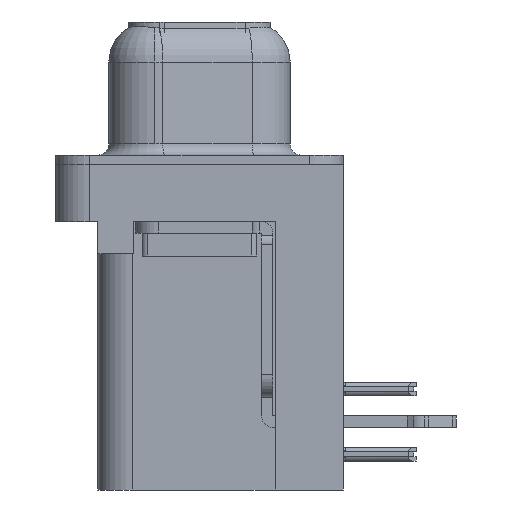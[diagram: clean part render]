
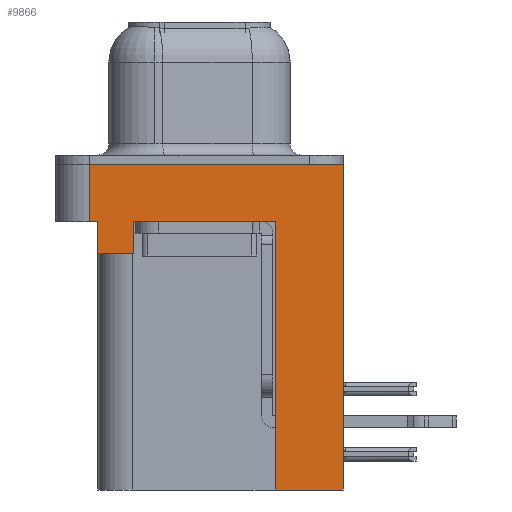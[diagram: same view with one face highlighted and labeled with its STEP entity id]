
A CAD part, left-side view. The second image highlights one B-rep face of the part: STEP entity #9866.
In plain terms, the highlighted planar face has unit normal (-1, 0, 0).
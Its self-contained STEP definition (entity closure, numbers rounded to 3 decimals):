
#662 = ORIENTED_EDGE ( 'NONE', *, *, #22296, .F. ) ;
#975 = CARTESIAN_POINT ( 'NONE',  ( -2.91, -3.295, -14.2 ) ) ;
#1129 = ORIENTED_EDGE ( 'NONE', *, *, #33008, .F. ) ;
#1270 = VECTOR ( 'NONE', #12453, 1000. ) ;
#1343 = EDGE_CURVE ( 'NONE', #36206, #31903, #29630, .T. ) ;
#2132 = LINE ( 'NONE', #27914, #9088 ) ;
#2595 = CARTESIAN_POINT ( 'NONE',  ( -2.91, -6.275, -14.2 ) ) ;
#2701 = EDGE_CURVE ( 'NONE', #25302, #26912, #2132, .T. ) ;
#2779 = CARTESIAN_POINT ( 'NONE',  ( -2.91, -3.295, -14.2 ) ) ;
#3863 = DIRECTION ( 'NONE',  ( 0., 0., 1. ) ) ;
#4467 = LINE ( 'NONE', #21187, #1270 ) ;
#5905 = LINE ( 'NONE', #31322, #26976 ) ;
#6474 = ORIENTED_EDGE ( 'NONE', *, *, #16695, .F. ) ;
#7933 = CARTESIAN_POINT ( 'NONE',  ( -2.91, -3.295, -2.5 ) ) ;
#8213 = CARTESIAN_POINT ( 'NONE',  ( -2.91, 4.775, -2.5 ) ) ;
#8219 = DIRECTION ( 'NONE',  ( 0., 0., 1. ) ) ;
#8306 = CARTESIAN_POINT ( 'NONE',  ( -2.91, 4.425, -3.9 ) ) ;
#8518 = ORIENTED_EDGE ( 'NONE', *, *, #31069, .F. ) ;
#8621 = DIRECTION ( 'NONE',  ( 0., 0., 1. ) ) ;
#8640 = EDGE_LOOP ( 'NONE', ( #11275, #8518, #35854, #1129, #662, #28178, #12209, #31163, #6474, #33613 ) ) ;
#8813 = LINE ( 'NONE', #14006, #20465 ) ;
#8950 = LINE ( 'NONE', #975, #25803 ) ;
#8978 = DIRECTION ( 'NONE',  ( 0., 0., 1. ) ) ;
#9088 = VECTOR ( 'NONE', #36262, 1000. ) ;
#9105 = VERTEX_POINT ( 'NONE', #32673 ) ;
#9159 = EDGE_CURVE ( 'NONE', #9105, #36573, #4467, .T. ) ;
#9362 = VECTOR ( 'NONE', #3863, 1000. ) ;
#9866 = ADVANCED_FACE ( 'NONE', ( #32183 ), #26425, .T. ) ;
#10618 = VERTEX_POINT ( 'NONE', #2779 ) ;
#11275 = ORIENTED_EDGE ( 'NONE', *, *, #1343, .F. ) ;
#12209 = ORIENTED_EDGE ( 'NONE', *, *, #9159, .T. ) ;
#12453 = DIRECTION ( 'NONE',  ( 0., -1., 0. ) ) ;
#12659 = VECTOR ( 'NONE', #35088, 1000. ) ;
#12745 = CARTESIAN_POINT ( 'NONE',  ( -2.91, -3.295, -14.2 ) ) ;
#13602 = EDGE_CURVE ( 'NONE', #10618, #36573, #17797, .T. ) ;
#13910 = CARTESIAN_POINT ( 'NONE',  ( -2.91, 4.425, -2.5 ) ) ;
#14006 = CARTESIAN_POINT ( 'NONE',  ( -2.91, 4.425, -3.9 ) ) ;
#14107 = VECTOR ( 'NONE', #20742, 1000. ) ;
#14548 = CARTESIAN_POINT ( 'NONE',  ( -2.91, -6.275, -2.5 ) ) ;
#15465 = VERTEX_POINT ( 'NONE', #28028 ) ;
#16290 = EDGE_CURVE ( 'NONE', #36254, #31903, #5905, .T. ) ;
#16695 = EDGE_CURVE ( 'NONE', #36254, #10618, #8950, .T. ) ;
#17797 = LINE ( 'NONE', #12745, #9362 ) ;
#18054 = LINE ( 'NONE', #20830, #12659 ) ;
#18504 = AXIS2_PLACEMENT_3D ( 'NONE', #14548, #26612, #8978 ) ;
#18789 = VECTOR ( 'NONE', #8219, 1000. ) ;
#20465 = VECTOR ( 'NONE', #8621, 1000. ) ;
#20569 = DIRECTION ( 'NONE',  ( 0., 0., 1. ) ) ;
#20742 = DIRECTION ( 'NONE',  ( 0., -1., 0. ) ) ;
#20830 = CARTESIAN_POINT ( 'NONE',  ( -2.91, 4.775, -2.5 ) ) ;
#21187 = CARTESIAN_POINT ( 'NONE',  ( -2.91, -6.275, -2.5 ) ) ;
#21754 = CARTESIAN_POINT ( 'NONE',  ( -2.91, 4.425, -3.9 ) ) ;
#22296 = EDGE_CURVE ( 'NONE', #15465, #29057, #30947, .T. ) ;
#22421 = DIRECTION ( 'NONE',  ( 0., 1., 0. ) ) ;
#23803 = DIRECTION ( 'NONE',  ( 0., 1., 0. ) ) ;
#25302 = VERTEX_POINT ( 'NONE', #8213 ) ;
#25803 = VECTOR ( 'NONE', #23803, 1000. ) ;
#26387 = EDGE_CURVE ( 'NONE', #15465, #9105, #30689, .T. ) ;
#26425 = PLANE ( 'NONE',  #18504 ) ;
#26612 = DIRECTION ( 'NONE',  ( -1., 0., 0. ) ) ;
#26912 = VERTEX_POINT ( 'NONE', #13910 ) ;
#26976 = VECTOR ( 'NONE', #20569, 1000. ) ;
#27166 = CARTESIAN_POINT ( 'NONE',  ( -2.91, 2.895, -3.9 ) ) ;
#27914 = CARTESIAN_POINT ( 'NONE',  ( -2.91, -6.275, -2.5 ) ) ;
#28028 = CARTESIAN_POINT ( 'NONE',  ( -2.91, 2.895, -3.9 ) ) ;
#28178 = ORIENTED_EDGE ( 'NONE', *, *, #26387, .T. ) ;
#29057 = VERTEX_POINT ( 'NONE', #21754 ) ;
#29363 = CARTESIAN_POINT ( 'NONE',  ( -2.91, -6.275, 0. ) ) ;
#29630 = LINE ( 'NONE', #32591, #14107 ) ;
#30689 = LINE ( 'NONE', #27166, #18789 ) ;
#30947 = LINE ( 'NONE', #8306, #33452 ) ;
#31069 = EDGE_CURVE ( 'NONE', #25302, #36206, #18054, .T. ) ;
#31163 = ORIENTED_EDGE ( 'NONE', *, *, #13602, .F. ) ;
#31322 = CARTESIAN_POINT ( 'NONE',  ( -2.91, -6.275, -2.5 ) ) ;
#31903 = VERTEX_POINT ( 'NONE', #29363 ) ;
#32183 = FACE_OUTER_BOUND ( 'NONE', #8640, .T. ) ;
#32591 = CARTESIAN_POINT ( 'NONE',  ( -2.91, -6.275, 0. ) ) ;
#32673 = CARTESIAN_POINT ( 'NONE',  ( -2.91, 2.895, -2.5 ) ) ;
#33008 = EDGE_CURVE ( 'NONE', #29057, #26912, #8813, .T. ) ;
#33452 = VECTOR ( 'NONE', #22421, 1000. ) ;
#33613 = ORIENTED_EDGE ( 'NONE', *, *, #16290, .T. ) ;
#35088 = DIRECTION ( 'NONE',  ( 0., 0., 1. ) ) ;
#35854 = ORIENTED_EDGE ( 'NONE', *, *, #2701, .T. ) ;
#36183 = CARTESIAN_POINT ( 'NONE',  ( -2.91, 4.775, 0. ) ) ;
#36206 = VERTEX_POINT ( 'NONE', #36183 ) ;
#36254 = VERTEX_POINT ( 'NONE', #2595 ) ;
#36262 = DIRECTION ( 'NONE',  ( 0., -1., 0. ) ) ;
#36573 = VERTEX_POINT ( 'NONE', #7933 ) ;
